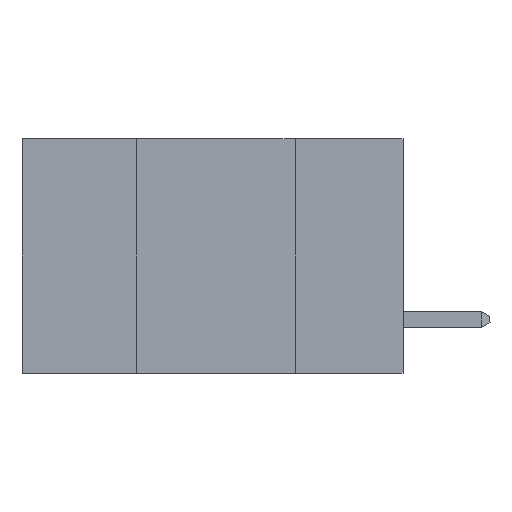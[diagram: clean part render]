
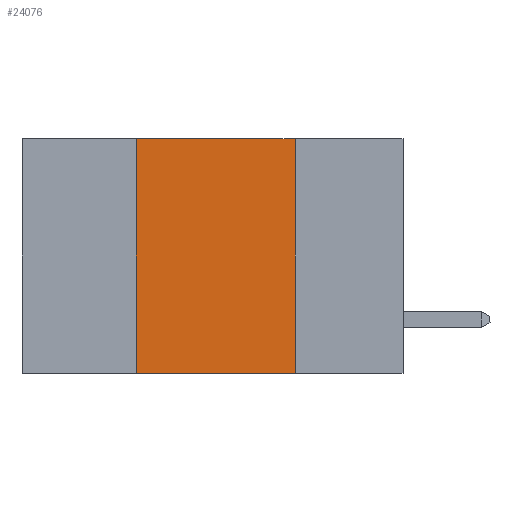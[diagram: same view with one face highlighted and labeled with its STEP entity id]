
A CAD part, left-side view. The second image highlights one B-rep face of the part: STEP entity #24076.
In plain terms, the highlighted planar face has unit normal (-1, 0, 0).
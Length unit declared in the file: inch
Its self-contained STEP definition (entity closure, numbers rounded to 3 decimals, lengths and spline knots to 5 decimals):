
#1768 = LINE ( 'NONE', #14088, #18018 ) ;
#3073 = VERTEX_POINT ( 'NONE', #25407 ) ;
#3890 = VECTOR ( 'NONE', #16323, 39.37008 ) ;
#3921 = CARTESIAN_POINT ( 'NONE',  ( 0., 0.6, 0. ) ) ;
#4294 = EDGE_CURVE ( 'NONE', #3073, #12404, #1768, .T. ) ;
#4664 = FACE_OUTER_BOUND ( 'NONE', #18724, .T. ) ;
#6018 = VECTOR ( 'NONE', #21507, 39.37008 ) ;
#6153 = CARTESIAN_POINT ( 'NONE',  ( 0., 0.42, 0. ) ) ;
#8092 = EDGE_CURVE ( 'NONE', #25045, #3073, #17668, .T. ) ;
#8410 = DIRECTION ( 'NONE',  ( 1., 0., 0. ) ) ;
#9766 = CARTESIAN_POINT ( 'NONE',  ( 0., 0.17, -0.37 ) ) ;
#10055 = VECTOR ( 'NONE', #26540, 39.37008 ) ;
#12404 = VERTEX_POINT ( 'NONE', #24065 ) ;
#12781 = PLANE ( 'NONE',  #13978 ) ;
#13978 = AXIS2_PLACEMENT_3D ( 'NONE', #3921, #8410, #23770 ) ;
#14088 = CARTESIAN_POINT ( 'NONE',  ( 0., 0.6, 0. ) ) ;
#14650 = ORIENTED_EDGE ( 'NONE', *, *, #4294, .F. ) ;
#15305 = ORIENTED_EDGE ( 'NONE', *, *, #8092, .F. ) ;
#16323 = DIRECTION ( 'NONE',  ( 0., 0., -1. ) ) ;
#16344 = LINE ( 'NONE', #20639, #3890 ) ;
#17668 = LINE ( 'NONE', #6153, #6018 ) ;
#18018 = VECTOR ( 'NONE', #27151, 39.37008 ) ;
#18724 = EDGE_LOOP ( 'NONE', ( #25588, #14650, #15305, #26950 ) ) ;
#18928 = EDGE_CURVE ( 'NONE', #25045, #28363, #21690, .T. ) ;
#20639 = CARTESIAN_POINT ( 'NONE',  ( 0., 0.17, 0. ) ) ;
#21507 = DIRECTION ( 'NONE',  ( 0., 0., 1. ) ) ;
#21690 = LINE ( 'NONE', #24321, #10055 ) ;
#22574 = CARTESIAN_POINT ( 'NONE',  ( 0., 0.42, -0.37 ) ) ;
#22818 = EDGE_CURVE ( 'NONE', #12404, #28363, #16344, .T. ) ;
#23770 = DIRECTION ( 'NONE',  ( 0., 0., -1. ) ) ;
#24065 = CARTESIAN_POINT ( 'NONE',  ( 0., 0.17, 0. ) ) ;
#24076 = ADVANCED_FACE ( 'NONE', ( #4664 ), #12781, .F. ) ;
#24321 = CARTESIAN_POINT ( 'NONE',  ( 0., 0.6, -0.37 ) ) ;
#25045 = VERTEX_POINT ( 'NONE', #22574 ) ;
#25407 = CARTESIAN_POINT ( 'NONE',  ( 0., 0.42, 0. ) ) ;
#25588 = ORIENTED_EDGE ( 'NONE', *, *, #22818, .F. ) ;
#26540 = DIRECTION ( 'NONE',  ( 0., -1., 0. ) ) ;
#26950 = ORIENTED_EDGE ( 'NONE', *, *, #18928, .T. ) ;
#27151 = DIRECTION ( 'NONE',  ( 0., -1., 0. ) ) ;
#28363 = VERTEX_POINT ( 'NONE', #9766 ) ;
